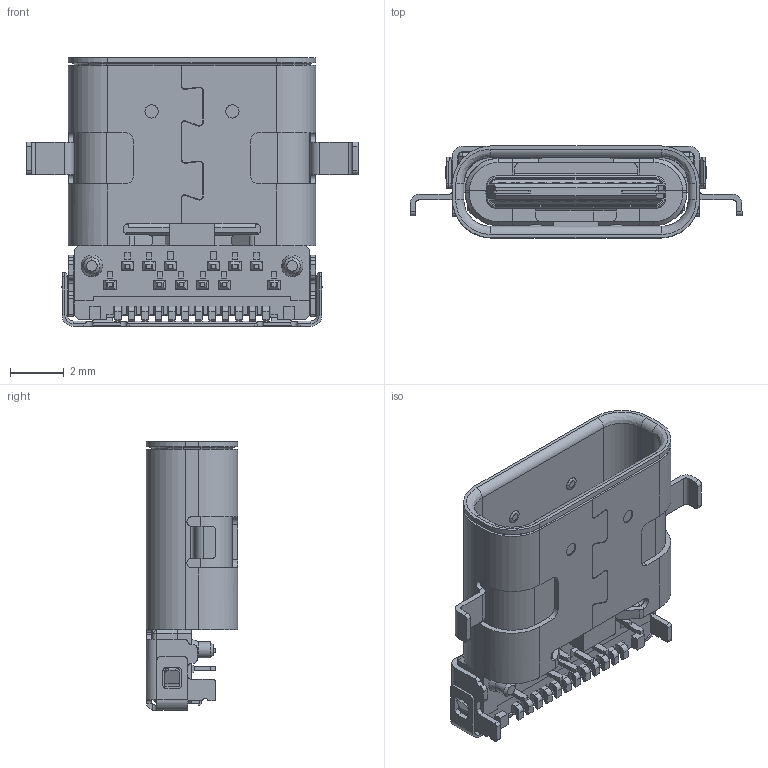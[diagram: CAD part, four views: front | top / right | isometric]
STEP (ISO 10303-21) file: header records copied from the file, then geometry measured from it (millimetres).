
FILE_DESCRIPTION (( 'STEP AP214' ), '1' );
FILE_NAME ('698C124-215-211.STEP', '2021-01-15T18:28:52', ( '' ), ( '' ), 'SwSTEP 2.0', 'SolidWorks 2020', '' );
FILE_SCHEMA (( 'AUTOMOTIVE_DESIGN' ));
Length unit declared in the file: millimetre
Products named in the file (6): Shell3 698C124-X15-211; Shell2 698C124-X15-211; Shell1 698C124-X15-211; Insulator2 698C124-X15-211; Insulator1 698C124-X15-211; 698C124-215-211
Assembly tree (5 placements, depth 2):
  698C124-215-211
    Shell2 698C124-X15-211
    Shell1 698C124-X15-211
    Insulator1 698C124-X15-211
    Shell3 698C124-X15-211
    Insulator2 698C124-X15-211
Bounding box: 12.35 x 3.42 x 10 mm (x, y, z)
Volume: 137.1 mm3; surface area: 1245.4 mm2
Topology: 5 solids, 56 shells, 3308 faces, 9266 edges, 6067 vertices
Faces by surface type: plane 2468, cylinder 747, cone 56, bspline 37
Entity records: 113909 total; most frequent: CARTESIAN_POINT 21611, ORIENTED_EDGE 18520, DIRECTION 16739, EDGE_CURVE 9260, LINE 7319, VECTOR 7319, VERTEX_POINT 6067, AXIS2_PLACEMENT_3D 4710
